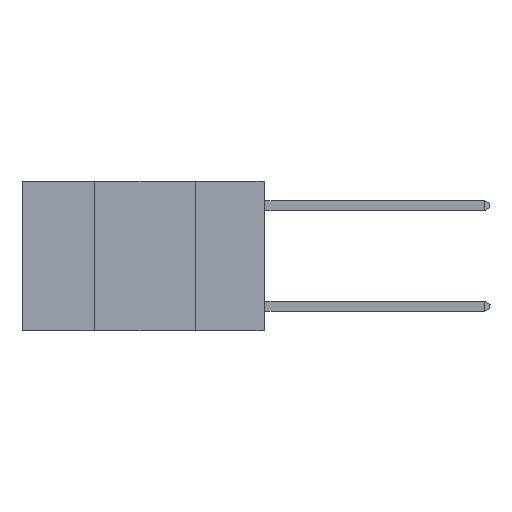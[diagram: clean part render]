
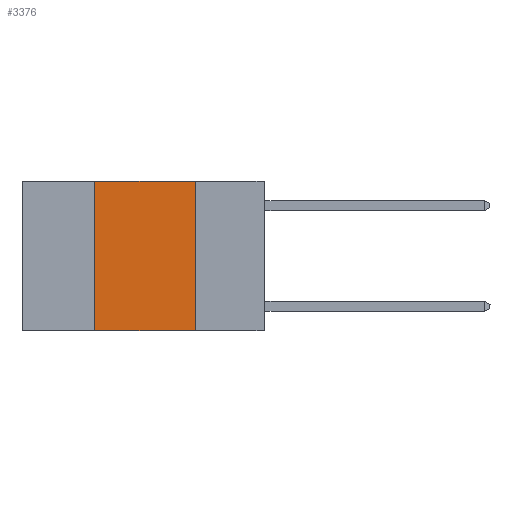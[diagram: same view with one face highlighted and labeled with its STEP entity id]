
A CAD part, left-side view. The second image highlights one B-rep face of the part: STEP entity #3376.
In plain terms, the highlighted planar face has unit normal (-1, 0, 0).
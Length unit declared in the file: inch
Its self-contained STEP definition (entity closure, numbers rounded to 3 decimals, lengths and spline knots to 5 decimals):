
#121 = CARTESIAN_POINT ( 'NONE',  ( 0., 0.42, 0. ) ) ;
#230 = ORIENTED_EDGE ( 'NONE', *, *, #6585, .F. ) ;
#891 = DIRECTION ( 'NONE',  ( 0., 0., 1. ) ) ;
#1024 = EDGE_CURVE ( 'NONE', #7806, #4858, #5246, .T. ) ;
#1224 = VECTOR ( 'NONE', #891, 39.37008 ) ;
#1420 = DIRECTION ( 'NONE',  ( 0., 0., -1. ) ) ;
#1783 = CARTESIAN_POINT ( 'NONE',  ( 0., 0.17, 0. ) ) ;
#2852 = PLANE ( 'NONE',  #7953 ) ;
#3254 = CARTESIAN_POINT ( 'NONE',  ( 0., 0.42, 0. ) ) ;
#3362 = VECTOR ( 'NONE', #8596, 39.37008 ) ;
#3376 = ADVANCED_FACE ( 'NONE', ( #5673 ), #2852, .F. ) ;
#3425 = VECTOR ( 'NONE', #5010, 39.37008 ) ;
#3538 = DIRECTION ( 'NONE',  ( 0., 0., -1. ) ) ;
#3628 = CARTESIAN_POINT ( 'NONE',  ( 0., 0.17, -0.37 ) ) ;
#3920 = EDGE_CURVE ( 'NONE', #4858, #8238, #7086, .T. ) ;
#3963 = CARTESIAN_POINT ( 'NONE',  ( 0., 0.42, -0.37 ) ) ;
#4083 = ORIENTED_EDGE ( 'NONE', *, *, #1024, .F. ) ;
#4308 = ORIENTED_EDGE ( 'NONE', *, *, #5976, .T. ) ;
#4395 = VERTEX_POINT ( 'NONE', #3963 ) ;
#4858 = VERTEX_POINT ( 'NONE', #1783 ) ;
#5010 = DIRECTION ( 'NONE',  ( 0., -1., 0. ) ) ;
#5246 = LINE ( 'NONE', #5553, #3362 ) ;
#5553 = CARTESIAN_POINT ( 'NONE',  ( 0., 0.6, 0. ) ) ;
#5638 = CARTESIAN_POINT ( 'NONE',  ( 0., 0.6, 0. ) ) ;
#5673 = FACE_OUTER_BOUND ( 'NONE', #8381, .T. ) ;
#5719 = CARTESIAN_POINT ( 'NONE',  ( 0., 0.6, -0.37 ) ) ;
#5976 = EDGE_CURVE ( 'NONE', #4395, #8238, #8930, .T. ) ;
#6585 = EDGE_CURVE ( 'NONE', #4395, #7806, #6710, .T. ) ;
#6710 = LINE ( 'NONE', #121, #1224 ) ;
#6935 = CARTESIAN_POINT ( 'NONE',  ( 0., 0.17, 0. ) ) ;
#7086 = LINE ( 'NONE', #6935, #8259 ) ;
#7394 = ORIENTED_EDGE ( 'NONE', *, *, #3920, .F. ) ;
#7732 = DIRECTION ( 'NONE',  ( 1., 0., 0. ) ) ;
#7806 = VERTEX_POINT ( 'NONE', #3254 ) ;
#7953 = AXIS2_PLACEMENT_3D ( 'NONE', #5638, #7732, #3538 ) ;
#8238 = VERTEX_POINT ( 'NONE', #3628 ) ;
#8259 = VECTOR ( 'NONE', #1420, 39.37008 ) ;
#8381 = EDGE_LOOP ( 'NONE', ( #7394, #4083, #230, #4308 ) ) ;
#8596 = DIRECTION ( 'NONE',  ( 0., -1., 0. ) ) ;
#8930 = LINE ( 'NONE', #5719, #3425 ) ;
